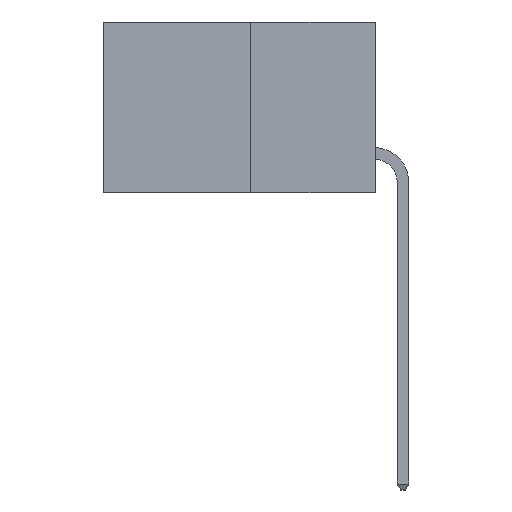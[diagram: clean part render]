
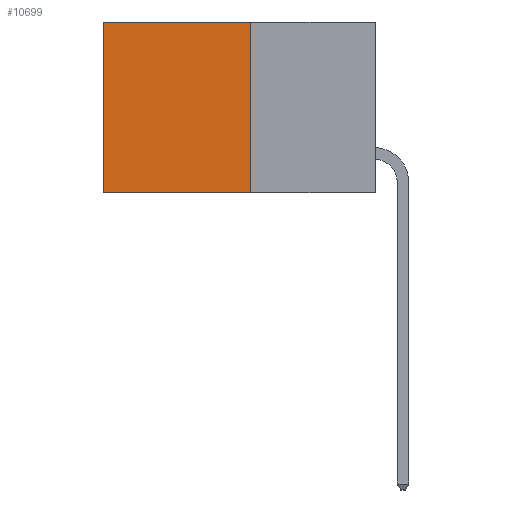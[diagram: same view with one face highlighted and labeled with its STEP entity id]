
A CAD part, left-side view. The second image highlights one B-rep face of the part: STEP entity #10699.
In plain terms, the highlighted planar face has unit normal (-1, 0, 0).
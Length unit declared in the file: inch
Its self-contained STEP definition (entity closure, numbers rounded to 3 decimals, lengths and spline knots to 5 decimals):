
#490 = LINE ( 'NONE', #4127, #9078 ) ;
#1444 = VERTEX_POINT ( 'NONE', #12886 ) ;
#1971 = VECTOR ( 'NONE', #13479, 39.37008 ) ;
#1993 = EDGE_CURVE ( 'NONE', #3293, #1444, #10379, .T. ) ;
#2204 = CARTESIAN_POINT ( 'NONE',  ( 0.277, 0.59, -0.37 ) ) ;
#3014 = EDGE_CURVE ( 'NONE', #7901, #1444, #490, .T. ) ;
#3035 = VERTEX_POINT ( 'NONE', #14062 ) ;
#3038 = LINE ( 'NONE', #13784, #1971 ) ;
#3195 = DIRECTION ( 'NONE',  ( 0., 0., -1. ) ) ;
#3245 = DIRECTION ( 'NONE',  ( 1., 0., 0. ) ) ;
#3293 = VERTEX_POINT ( 'NONE', #6035 ) ;
#3318 = CARTESIAN_POINT ( 'NONE',  ( 0.277, 0.27, -0.37 ) ) ;
#3370 = PLANE ( 'NONE',  #6659 ) ;
#3373 = ORIENTED_EDGE ( 'NONE', *, *, #5942, .T. ) ;
#3885 = VECTOR ( 'NONE', #13982, 39.37008 ) ;
#4127 = CARTESIAN_POINT ( 'NONE',  ( 0.277, 0.27, -0.37 ) ) ;
#5059 = DIRECTION ( 'NONE',  ( 0., 1., 0. ) ) ;
#5920 = DIRECTION ( 'NONE',  ( 0., 0., -1. ) ) ;
#5942 = EDGE_CURVE ( 'NONE', #3035, #3293, #7193, .T. ) ;
#6035 = CARTESIAN_POINT ( 'NONE',  ( 0.277, 0.59, 0. ) ) ;
#6659 = AXIS2_PLACEMENT_3D ( 'NONE', #3318, #3245, #3195 ) ;
#7193 = LINE ( 'NONE', #13931, #3885 ) ;
#7901 = VERTEX_POINT ( 'NONE', #11681 ) ;
#8948 = ORIENTED_EDGE ( 'NONE', *, *, #3014, .F. ) ;
#9078 = VECTOR ( 'NONE', #5059, 39.37008 ) ;
#10379 = LINE ( 'NONE', #2204, #10692 ) ;
#10692 = VECTOR ( 'NONE', #5920, 39.37008 ) ;
#10699 = ADVANCED_FACE ( 'NONE', ( #11876 ), #3370, .F. ) ;
#11334 = ORIENTED_EDGE ( 'NONE', *, *, #1993, .T. ) ;
#11386 = EDGE_CURVE ( 'NONE', #3035, #7901, #3038, .T. ) ;
#11653 = ORIENTED_EDGE ( 'NONE', *, *, #11386, .F. ) ;
#11681 = CARTESIAN_POINT ( 'NONE',  ( 0.277, 0.27, -0.37 ) ) ;
#11876 = FACE_OUTER_BOUND ( 'NONE', #12223, .T. ) ;
#12223 = EDGE_LOOP ( 'NONE', ( #11334, #8948, #11653, #3373 ) ) ;
#12886 = CARTESIAN_POINT ( 'NONE',  ( 0.277, 0.59, -0.37 ) ) ;
#13479 = DIRECTION ( 'NONE',  ( 0., 0., -1. ) ) ;
#13784 = CARTESIAN_POINT ( 'NONE',  ( 0.277, 0.27, -0.37 ) ) ;
#13931 = CARTESIAN_POINT ( 'NONE',  ( 0.277, 0.27, 0. ) ) ;
#13982 = DIRECTION ( 'NONE',  ( 0., 1., 0. ) ) ;
#14062 = CARTESIAN_POINT ( 'NONE',  ( 0.277, 0.27, 0. ) ) ;
